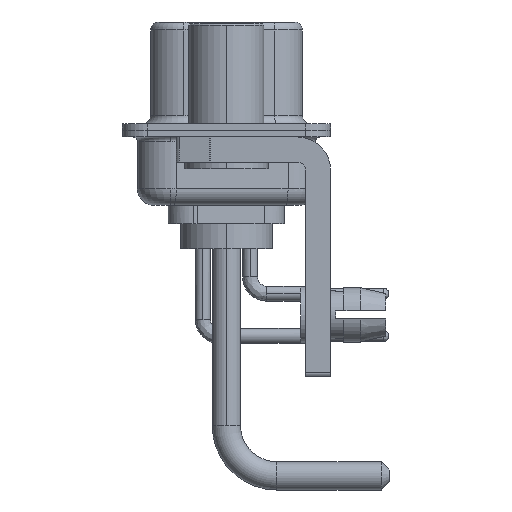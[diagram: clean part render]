
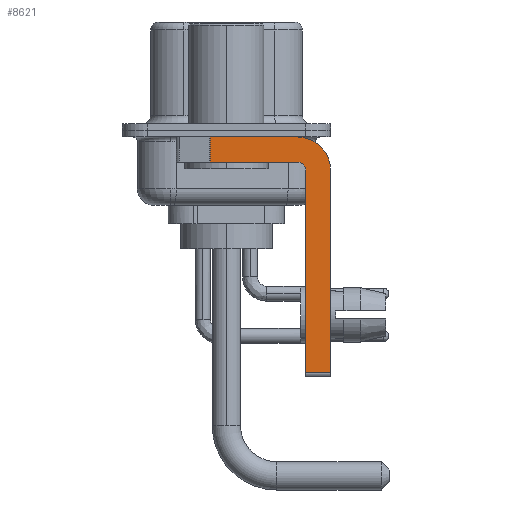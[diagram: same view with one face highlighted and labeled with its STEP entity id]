
A CAD part, left-side view. The second image highlights one B-rep face of the part: STEP entity #8621.
In plain terms, the highlighted planar face has unit normal (-1, 0, 0).
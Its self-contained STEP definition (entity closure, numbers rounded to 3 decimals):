
#73 = DIRECTION ( 'NONE',  ( 1., 0., 0. ) ) ;
#547 = CARTESIAN_POINT ( 'NONE',  ( -2.9, -6.25, -14.55 ) ) ;
#945 = LINE ( 'NONE', #3050, #22986 ) ;
#1198 = ORIENTED_EDGE ( 'NONE', *, *, #20357, .F. ) ;
#1310 = CARTESIAN_POINT ( 'NONE',  ( -2.9, -6.25, -2.4 ) ) ;
#1534 = CIRCLE ( 'NONE', #11203, 0.5 ) ;
#1615 = EDGE_CURVE ( 'NONE', #25510, #16381, #2733, .T. ) ;
#1917 = DIRECTION ( 'NONE',  ( -1., 0., 0. ) ) ;
#1927 = DIRECTION ( 'NONE',  ( 0., 0., -1. ) ) ;
#2706 = ORIENTED_EDGE ( 'NONE', *, *, #14943, .F. ) ;
#2733 = LINE ( 'NONE', #14821, #18095 ) ;
#2781 = DIRECTION ( 'NONE',  ( 0., 0., -1. ) ) ;
#3050 = CARTESIAN_POINT ( 'NONE',  ( -2.9, 0.978, -1.9 ) ) ;
#3318 = ORIENTED_EDGE ( 'NONE', *, *, #20031, .F. ) ;
#3429 = ORIENTED_EDGE ( 'NONE', *, *, #11433, .T. ) ;
#4277 = DIRECTION ( 'NONE',  ( 0., 0., -1. ) ) ;
#5918 = VECTOR ( 'NONE', #6314, 1000. ) ;
#6263 = CARTESIAN_POINT ( 'NONE',  ( -2.9, -4.25, -2.4 ) ) ;
#6314 = DIRECTION ( 'NONE',  ( 0., 1., 0. ) ) ;
#6987 = VERTEX_POINT ( 'NONE', #17835 ) ;
#7294 = ORIENTED_EDGE ( 'NONE', *, *, #15944, .F. ) ;
#7832 = VECTOR ( 'NONE', #1927, 1000. ) ;
#7971 = DIRECTION ( 'NONE',  ( 0., 0., 1. ) ) ;
#8410 = CARTESIAN_POINT ( 'NONE',  ( -2.9, -4.25, -1.9 ) ) ;
#8621 = ADVANCED_FACE ( 'NONE', ( #16799 ), #24823, .F. ) ;
#9302 = CARTESIAN_POINT ( 'NONE',  ( -2.9, 3., -0.4 ) ) ;
#9428 = CARTESIAN_POINT ( 'NONE',  ( -2.9, 0.978, -1.9 ) ) ;
#9965 = CARTESIAN_POINT ( 'NONE',  ( -2.9, -4.75, -2.4 ) ) ;
#9973 = VERTEX_POINT ( 'NONE', #9428 ) ;
#10484 = VERTEX_POINT ( 'NONE', #11018 ) ;
#10571 = CARTESIAN_POINT ( 'NONE',  ( -2.9, -4.25, -2.4 ) ) ;
#10572 = EDGE_CURVE ( 'NONE', #6987, #10484, #21515, .T. ) ;
#10878 = CARTESIAN_POINT ( 'NONE',  ( -2.9, -4.25, -2.4 ) ) ;
#11018 = CARTESIAN_POINT ( 'NONE',  ( -2.9, -4.25, -0.4 ) ) ;
#11203 = AXIS2_PLACEMENT_3D ( 'NONE', #6263, #1917, #7971 ) ;
#11404 = CARTESIAN_POINT ( 'NONE',  ( -2.9, -4.75, -14.8 ) ) ;
#11433 = EDGE_CURVE ( 'NONE', #6987, #9973, #945, .T. ) ;
#13385 = DIRECTION ( 'NONE',  ( 0., 0., 1. ) ) ;
#13632 = CARTESIAN_POINT ( 'NONE',  ( -2.9, -6.25, -2.4 ) ) ;
#14821 = CARTESIAN_POINT ( 'NONE',  ( -2.9, -4.25, -14.55 ) ) ;
#14943 = EDGE_CURVE ( 'NONE', #15314, #16381, #19940, .T. ) ;
#15314 = VERTEX_POINT ( 'NONE', #1310 ) ;
#15737 = DIRECTION ( 'NONE',  ( 0., -1., 0. ) ) ;
#15944 = EDGE_CURVE ( 'NONE', #10484, #15314, #19613, .T. ) ;
#16381 = VERTEX_POINT ( 'NONE', #547 ) ;
#16433 = LINE ( 'NONE', #8410, #5918 ) ;
#16799 = FACE_OUTER_BOUND ( 'NONE', #24032, .T. ) ;
#16923 = DIRECTION ( 'NONE',  ( 0., 0., -1. ) ) ;
#17441 = AXIS2_PLACEMENT_3D ( 'NONE', #10878, #18899, #16923 ) ;
#17548 = VECTOR ( 'NONE', #15737, 1000. ) ;
#17790 = ORIENTED_EDGE ( 'NONE', *, *, #1615, .T. ) ;
#17824 = ORIENTED_EDGE ( 'NONE', *, *, #25408, .F. ) ;
#17835 = CARTESIAN_POINT ( 'NONE',  ( -2.9, 0.978, -0.4 ) ) ;
#17850 = LINE ( 'NONE', #11404, #19720 ) ;
#18095 = VECTOR ( 'NONE', #24824, 1000. ) ;
#18370 = AXIS2_PLACEMENT_3D ( 'NONE', #10571, #73, #4277 ) ;
#18899 = DIRECTION ( 'NONE',  ( 1., 0., 0. ) ) ;
#19613 = CIRCLE ( 'NONE', #18370, 2. ) ;
#19720 = VECTOR ( 'NONE', #13385, 1000. ) ;
#19940 = LINE ( 'NONE', #13632, #7832 ) ;
#20031 = EDGE_CURVE ( 'NONE', #23319, #9973, #16433, .T. ) ;
#20357 = EDGE_CURVE ( 'NONE', #25510, #23209, #17850, .T. ) ;
#20467 = CARTESIAN_POINT ( 'NONE',  ( -2.9, -4.25, -1.9 ) ) ;
#21515 = LINE ( 'NONE', #9302, #17548 ) ;
#21565 = ORIENTED_EDGE ( 'NONE', *, *, #10572, .F. ) ;
#22986 = VECTOR ( 'NONE', #2781, 1000. ) ;
#23209 = VERTEX_POINT ( 'NONE', #9965 ) ;
#23319 = VERTEX_POINT ( 'NONE', #20467 ) ;
#24032 = EDGE_LOOP ( 'NONE', ( #21565, #3429, #3318, #17824, #1198, #17790, #2706, #7294 ) ) ;
#24404 = CARTESIAN_POINT ( 'NONE',  ( -2.9, -4.75, -14.55 ) ) ;
#24823 = PLANE ( 'NONE',  #17441 ) ;
#24824 = DIRECTION ( 'NONE',  ( 0., -1., 0. ) ) ;
#25408 = EDGE_CURVE ( 'NONE', #23209, #23319, #1534, .T. ) ;
#25510 = VERTEX_POINT ( 'NONE', #24404 ) ;
